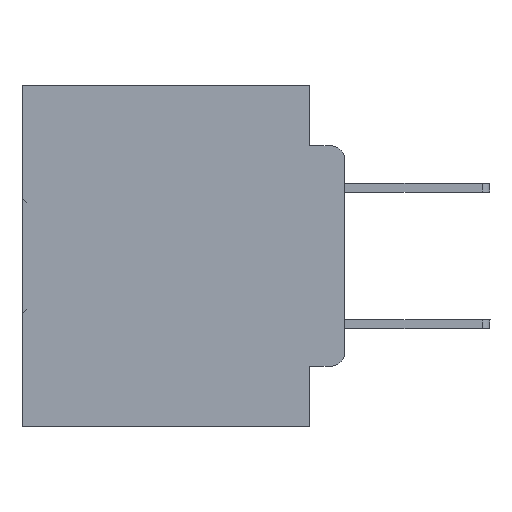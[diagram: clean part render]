
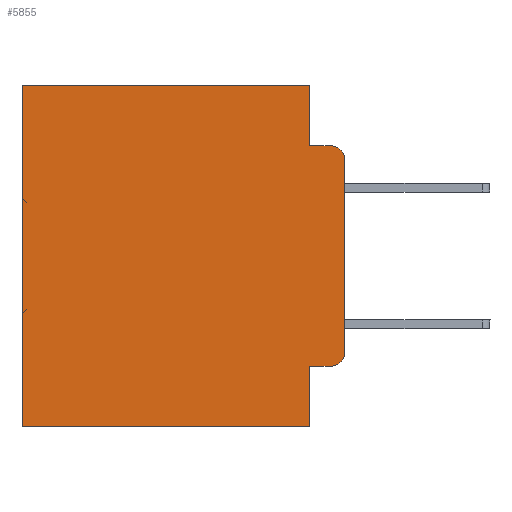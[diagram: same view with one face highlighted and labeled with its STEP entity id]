
A CAD part, left-side view. The second image highlights one B-rep face of the part: STEP entity #5855.
In plain terms, the highlighted planar face has unit normal (-1, 0, 0).
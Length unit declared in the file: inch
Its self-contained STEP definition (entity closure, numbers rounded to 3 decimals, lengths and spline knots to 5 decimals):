
#645 = AXIS2_PLACEMENT_3D ( 'NONE', #9615, #26787, #33952 ) ;
#894 = ORIENTED_EDGE ( 'NONE', *, *, #16018, .F. ) ;
#1244 = DIRECTION ( 'NONE',  ( 0., -1., 0. ) ) ;
#1390 = CARTESIAN_POINT ( 'NONE',  ( 0.298, 0.473, -0.5 ) ) ;
#2327 = EDGE_CURVE ( 'NONE', #10647, #5820, #7939, .T. ) ;
#2439 = LINE ( 'NONE', #13364, #9098 ) ;
#2599 = CARTESIAN_POINT ( 'NONE',  ( 0.298, 0.473, 0. ) ) ;
#2609 = EDGE_CURVE ( 'NONE', #20484, #25703, #20689, .T. ) ;
#2907 = CARTESIAN_POINT ( 'NONE',  ( 0.298, 0.051, 0. ) ) ;
#3879 = AXIS2_PLACEMENT_3D ( 'NONE', #13679, #33158, #16507 ) ;
#4465 = ORIENTED_EDGE ( 'NONE', *, *, #17891, .T. ) ;
#4519 = EDGE_LOOP ( 'NONE', ( #15486, #10033, #16369, #28123, #19012, #29868, #24271, #894, #17701, #4465 ) ) ;
#4722 = EDGE_CURVE ( 'NONE', #32012, #14476, #20969, .T. ) ;
#5820 = VERTEX_POINT ( 'NONE', #13099 ) ;
#5855 = ADVANCED_FACE ( 'NONE', ( #8618 ), #18281, .F. ) ;
#5989 = VECTOR ( 'NONE', #14633, 39.37008 ) ;
#6071 = VERTEX_POINT ( 'NONE', #20524 ) ;
#6483 = DIRECTION ( 'NONE',  ( 1., 0., 0. ) ) ;
#6720 = DIRECTION ( 'NONE',  ( 0., 0., -1. ) ) ;
#6863 = EDGE_CURVE ( 'NONE', #10647, #23268, #21758, .T. ) ;
#7124 = CIRCLE ( 'NONE', #3879, 0.02 ) ;
#7257 = LINE ( 'NONE', #28042, #21340 ) ;
#7537 = CARTESIAN_POINT ( 'NONE',  ( 0.298, 0.051, -0.4115 ) ) ;
#7663 = DIRECTION ( 'NONE',  ( 0., -1., 0. ) ) ;
#7939 = CIRCLE ( 'NONE', #645, 0.02 ) ;
#8122 = AXIS2_PLACEMENT_3D ( 'NONE', #32766, #6483, #6720 ) ;
#8618 = FACE_OUTER_BOUND ( 'NONE', #4519, .T. ) ;
#9098 = VECTOR ( 'NONE', #18907, 39.37008 ) ;
#9453 = EDGE_CURVE ( 'NONE', #33815, #14476, #2439, .T. ) ;
#9615 = CARTESIAN_POINT ( 'NONE',  ( 0.298, 0.02, -0.1085 ) ) ;
#10033 = ORIENTED_EDGE ( 'NONE', *, *, #2327, .T. ) ;
#10140 = CARTESIAN_POINT ( 'NONE',  ( 0.298, 0., 0. ) ) ;
#10555 = VECTOR ( 'NONE', #7663, 39.37008 ) ;
#10647 = VERTEX_POINT ( 'NONE', #35685 ) ;
#12494 = VECTOR ( 'NONE', #22406, 39.37008 ) ;
#13099 = CARTESIAN_POINT ( 'NONE',  ( 0.298, 0.02, -0.0885 ) ) ;
#13144 = EDGE_CURVE ( 'NONE', #20484, #32012, #23378, .T. ) ;
#13364 = CARTESIAN_POINT ( 'NONE',  ( 0.298, 0., -0.5 ) ) ;
#13391 = DIRECTION ( 'NONE',  ( 0., 0., -1. ) ) ;
#13660 = CARTESIAN_POINT ( 'NONE',  ( 0.298, 0.051, -0.4115 ) ) ;
#13679 = CARTESIAN_POINT ( 'NONE',  ( 0.298, 0.02, -0.3915 ) ) ;
#14138 = DIRECTION ( 'NONE',  ( 0., 0., -1. ) ) ;
#14476 = VERTEX_POINT ( 'NONE', #1390 ) ;
#14633 = DIRECTION ( 'NONE',  ( 0., 0., -1. ) ) ;
#15486 = ORIENTED_EDGE ( 'NONE', *, *, #6863, .F. ) ;
#16018 = EDGE_CURVE ( 'NONE', #22251, #33815, #7257, .T. ) ;
#16369 = ORIENTED_EDGE ( 'NONE', *, *, #18924, .F. ) ;
#16507 = DIRECTION ( 'NONE',  ( 0., 0., -1. ) ) ;
#17191 = VECTOR ( 'NONE', #1244, 39.37008 ) ;
#17701 = ORIENTED_EDGE ( 'NONE', *, *, #19768, .T. ) ;
#17891 = EDGE_CURVE ( 'NONE', #6071, #23268, #7124, .T. ) ;
#18028 = LINE ( 'NONE', #7537, #10555 ) ;
#18100 = LINE ( 'NONE', #34789, #17191 ) ;
#18281 = PLANE ( 'NONE',  #8122 ) ;
#18907 = DIRECTION ( 'NONE',  ( 0., 1., 0. ) ) ;
#18924 = EDGE_CURVE ( 'NONE', #25703, #5820, #18100, .T. ) ;
#19012 = ORIENTED_EDGE ( 'NONE', *, *, #13144, .T. ) ;
#19768 = EDGE_CURVE ( 'NONE', #22251, #6071, #18028, .T. ) ;
#19816 = CARTESIAN_POINT ( 'NONE',  ( 0.298, 0., -0.3915 ) ) ;
#20484 = VERTEX_POINT ( 'NONE', #2907 ) ;
#20524 = CARTESIAN_POINT ( 'NONE',  ( 0.298, 0.02, -0.4115 ) ) ;
#20689 = LINE ( 'NONE', #30762, #35403 ) ;
#20969 = LINE ( 'NONE', #26699, #5989 ) ;
#21340 = VECTOR ( 'NONE', #14138, 39.37008 ) ;
#21758 = LINE ( 'NONE', #10140, #12494 ) ;
#22251 = VERTEX_POINT ( 'NONE', #13660 ) ;
#22406 = DIRECTION ( 'NONE',  ( 0., 0., -1. ) ) ;
#23268 = VERTEX_POINT ( 'NONE', #19816 ) ;
#23378 = LINE ( 'NONE', #26643, #30711 ) ;
#24271 = ORIENTED_EDGE ( 'NONE', *, *, #9453, .F. ) ;
#25598 = CARTESIAN_POINT ( 'NONE',  ( 0.298, 0.051, -0.0885 ) ) ;
#25703 = VERTEX_POINT ( 'NONE', #25598 ) ;
#26643 = CARTESIAN_POINT ( 'NONE',  ( 0.298, 0., 0. ) ) ;
#26699 = CARTESIAN_POINT ( 'NONE',  ( 0.298, 0.473, 0. ) ) ;
#26787 = DIRECTION ( 'NONE',  ( -1., 0., 0. ) ) ;
#28042 = CARTESIAN_POINT ( 'NONE',  ( 0.298, 0.051, 0. ) ) ;
#28123 = ORIENTED_EDGE ( 'NONE', *, *, #2609, .F. ) ;
#28331 = CARTESIAN_POINT ( 'NONE',  ( 0.298, 0.051, -0.5 ) ) ;
#29868 = ORIENTED_EDGE ( 'NONE', *, *, #4722, .T. ) ;
#30711 = VECTOR ( 'NONE', #35011, 39.37008 ) ;
#30762 = CARTESIAN_POINT ( 'NONE',  ( 0.298, 0.051, 0. ) ) ;
#32012 = VERTEX_POINT ( 'NONE', #2599 ) ;
#32766 = CARTESIAN_POINT ( 'NONE',  ( 0.298, 0., 0. ) ) ;
#33158 = DIRECTION ( 'NONE',  ( -1., 0., 0. ) ) ;
#33815 = VERTEX_POINT ( 'NONE', #28331 ) ;
#33952 = DIRECTION ( 'NONE',  ( 0., 0., -1. ) ) ;
#34789 = CARTESIAN_POINT ( 'NONE',  ( 0.298, 0.051, -0.0885 ) ) ;
#35011 = DIRECTION ( 'NONE',  ( 0., 1., 0. ) ) ;
#35403 = VECTOR ( 'NONE', #13391, 39.37008 ) ;
#35685 = CARTESIAN_POINT ( 'NONE',  ( 0.298, 0., -0.1085 ) ) ;
